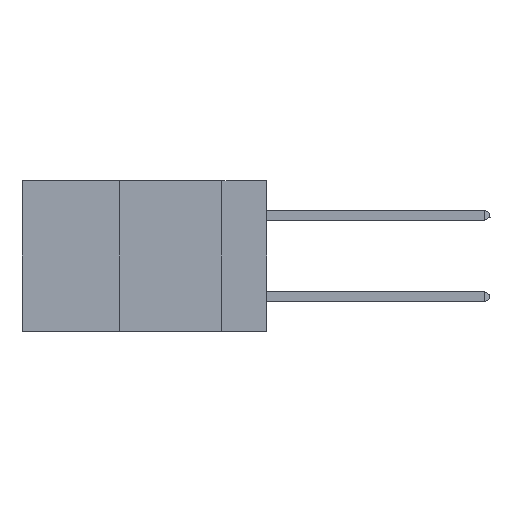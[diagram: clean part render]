
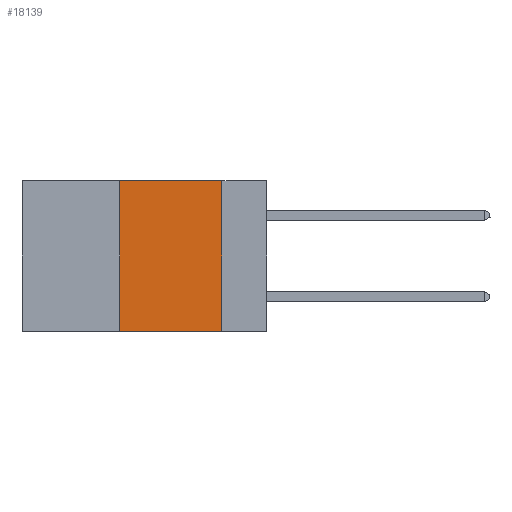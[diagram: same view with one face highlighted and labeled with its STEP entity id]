
A CAD part, left-side view. The second image highlights one B-rep face of the part: STEP entity #18139.
In plain terms, the highlighted planar face has unit normal (-1, 0, 0).
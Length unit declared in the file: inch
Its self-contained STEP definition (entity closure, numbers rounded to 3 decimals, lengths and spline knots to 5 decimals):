
#91 = PLANE ( 'NONE',  #18566 ) ;
#239 = ORIENTED_EDGE ( 'NONE', *, *, #8038, .F. ) ;
#277 = DIRECTION ( 'NONE',  ( 0., 0., -1. ) ) ;
#478 = CARTESIAN_POINT ( 'NONE',  ( 0., 0.11, 0. ) ) ;
#598 = FACE_OUTER_BOUND ( 'NONE', #3397, .T. ) ;
#1018 = CARTESIAN_POINT ( 'NONE',  ( 0., 0.36, 0. ) ) ;
#3397 = EDGE_LOOP ( 'NONE', ( #18714, #239, #12984, #15781 ) ) ;
#4132 = DIRECTION ( 'NONE',  ( 0., -1., 0. ) ) ;
#4984 = CARTESIAN_POINT ( 'NONE',  ( 0., 0.36, -0.37 ) ) ;
#5007 = LINE ( 'NONE', #7259, #15946 ) ;
#7254 = EDGE_CURVE ( 'NONE', #16905, #12823, #17442, .T. ) ;
#7259 = CARTESIAN_POINT ( 'NONE',  ( 0., 0.6, 0. ) ) ;
#7526 = CARTESIAN_POINT ( 'NONE',  ( 0., 0.36, 0. ) ) ;
#8038 = EDGE_CURVE ( 'NONE', #19170, #16905, #5007, .T. ) ;
#8798 = CARTESIAN_POINT ( 'NONE',  ( 0., 0.11, -0.37 ) ) ;
#9790 = DIRECTION ( 'NONE',  ( 0., 0., -1. ) ) ;
#11928 = VECTOR ( 'NONE', #4132, 39.37008 ) ;
#12575 = DIRECTION ( 'NONE',  ( 1., 0., 0. ) ) ;
#12823 = VERTEX_POINT ( 'NONE', #8798 ) ;
#12984 = ORIENTED_EDGE ( 'NONE', *, *, #17314, .F. ) ;
#13418 = CARTESIAN_POINT ( 'NONE',  ( 0., 0.6, -0.37 ) ) ;
#13447 = DIRECTION ( 'NONE',  ( 0., -1., 0. ) ) ;
#13625 = LINE ( 'NONE', #13418, #11928 ) ;
#13929 = CARTESIAN_POINT ( 'NONE',  ( 0., 0.11, 0. ) ) ;
#15773 = EDGE_CURVE ( 'NONE', #19382, #12823, #13625, .T. ) ;
#15781 = ORIENTED_EDGE ( 'NONE', *, *, #15773, .T. ) ;
#15946 = VECTOR ( 'NONE', #13447, 39.37008 ) ;
#16221 = VECTOR ( 'NONE', #9790, 39.37008 ) ;
#16905 = VERTEX_POINT ( 'NONE', #13929 ) ;
#16928 = LINE ( 'NONE', #7526, #18407 ) ;
#17207 = CARTESIAN_POINT ( 'NONE',  ( 0., 0.6, 0. ) ) ;
#17314 = EDGE_CURVE ( 'NONE', #19382, #19170, #16928, .T. ) ;
#17442 = LINE ( 'NONE', #478, #16221 ) ;
#18139 = ADVANCED_FACE ( 'NONE', ( #598 ), #91, .F. ) ;
#18407 = VECTOR ( 'NONE', #18658, 39.37008 ) ;
#18566 = AXIS2_PLACEMENT_3D ( 'NONE', #17207, #12575, #277 ) ;
#18658 = DIRECTION ( 'NONE',  ( 0., 0., 1. ) ) ;
#18714 = ORIENTED_EDGE ( 'NONE', *, *, #7254, .F. ) ;
#19170 = VERTEX_POINT ( 'NONE', #1018 ) ;
#19382 = VERTEX_POINT ( 'NONE', #4984 ) ;
